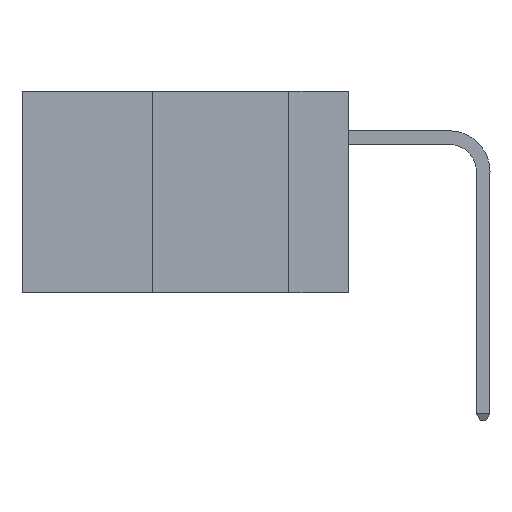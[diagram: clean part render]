
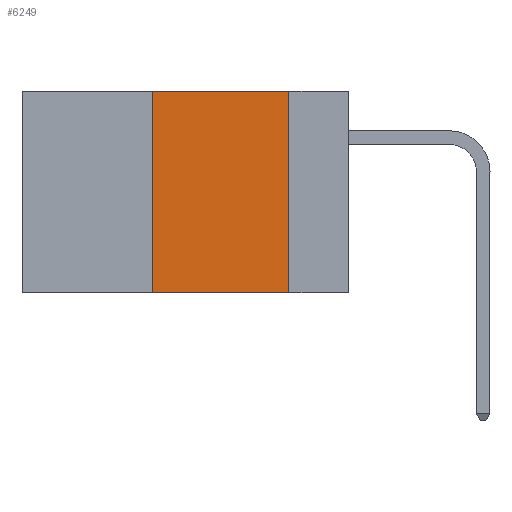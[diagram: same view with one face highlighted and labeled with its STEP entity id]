
A CAD part, left-side view. The second image highlights one B-rep face of the part: STEP entity #6249.
In plain terms, the highlighted planar face has unit normal (-1, 0, 0).
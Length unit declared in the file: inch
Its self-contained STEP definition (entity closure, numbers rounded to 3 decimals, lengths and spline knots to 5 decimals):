
#1501 = VECTOR ( 'NONE', #21089, 39.37008 ) ;
#1512 = EDGE_CURVE ( 'NONE', #12232, #7998, #13352, .T. ) ;
#2327 = CARTESIAN_POINT ( 'NONE',  ( 0., 0.6, -0.37 ) ) ;
#2422 = CARTESIAN_POINT ( 'NONE',  ( 0., 0.6, 0. ) ) ;
#5499 = DIRECTION ( 'NONE',  ( 0., 0., -1. ) ) ;
#6249 = ADVANCED_FACE ( 'NONE', ( #19995 ), #7720, .F. ) ;
#7720 = PLANE ( 'NONE',  #23847 ) ;
#7959 = CARTESIAN_POINT ( 'NONE',  ( 0., 0.11, -0.37 ) ) ;
#7998 = VERTEX_POINT ( 'NONE', #18802 ) ;
#8284 = VERTEX_POINT ( 'NONE', #7959 ) ;
#9321 = VERTEX_POINT ( 'NONE', #24479 ) ;
#9657 = ORIENTED_EDGE ( 'NONE', *, *, #19075, .F. ) ;
#11108 = EDGE_LOOP ( 'NONE', ( #9657, #13354, #12102, #24627 ) ) ;
#11282 = CARTESIAN_POINT ( 'NONE',  ( 0., 0.36, 0. ) ) ;
#12102 = ORIENTED_EDGE ( 'NONE', *, *, #1512, .F. ) ;
#12232 = VERTEX_POINT ( 'NONE', #17212 ) ;
#13352 = LINE ( 'NONE', #11282, #1501 ) ;
#13354 = ORIENTED_EDGE ( 'NONE', *, *, #20630, .F. ) ;
#13613 = DIRECTION ( 'NONE',  ( 0., 0., -1. ) ) ;
#13810 = VECTOR ( 'NONE', #5499, 39.37008 ) ;
#14032 = LINE ( 'NONE', #2422, #23211 ) ;
#17212 = CARTESIAN_POINT ( 'NONE',  ( 0., 0.36, -0.37 ) ) ;
#18127 = DIRECTION ( 'NONE',  ( 0., -1., 0. ) ) ;
#18295 = DIRECTION ( 'NONE',  ( 0., -1., 0. ) ) ;
#18802 = CARTESIAN_POINT ( 'NONE',  ( 0., 0.36, 0. ) ) ;
#19075 = EDGE_CURVE ( 'NONE', #9321, #8284, #24196, .T. ) ;
#19846 = VECTOR ( 'NONE', #18127, 39.37008 ) ;
#19995 = FACE_OUTER_BOUND ( 'NONE', #11108, .T. ) ;
#20554 = EDGE_CURVE ( 'NONE', #12232, #8284, #25028, .T. ) ;
#20630 = EDGE_CURVE ( 'NONE', #7998, #9321, #14032, .T. ) ;
#21089 = DIRECTION ( 'NONE',  ( 0., 0., 1. ) ) ;
#23211 = VECTOR ( 'NONE', #18295, 39.37008 ) ;
#23347 = CARTESIAN_POINT ( 'NONE',  ( 0., 0.6, 0. ) ) ;
#23847 = AXIS2_PLACEMENT_3D ( 'NONE', #23347, #25298, #13613 ) ;
#24196 = LINE ( 'NONE', #25019, #13810 ) ;
#24479 = CARTESIAN_POINT ( 'NONE',  ( 0., 0.11, 0. ) ) ;
#24627 = ORIENTED_EDGE ( 'NONE', *, *, #20554, .T. ) ;
#25019 = CARTESIAN_POINT ( 'NONE',  ( 0., 0.11, 0. ) ) ;
#25028 = LINE ( 'NONE', #2327, #19846 ) ;
#25298 = DIRECTION ( 'NONE',  ( 1., 0., 0. ) ) ;
